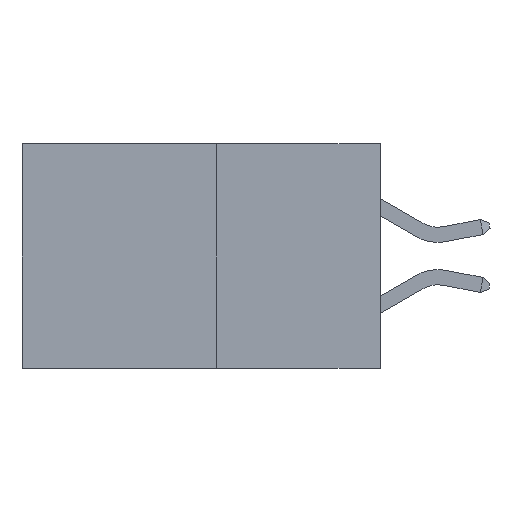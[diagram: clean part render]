
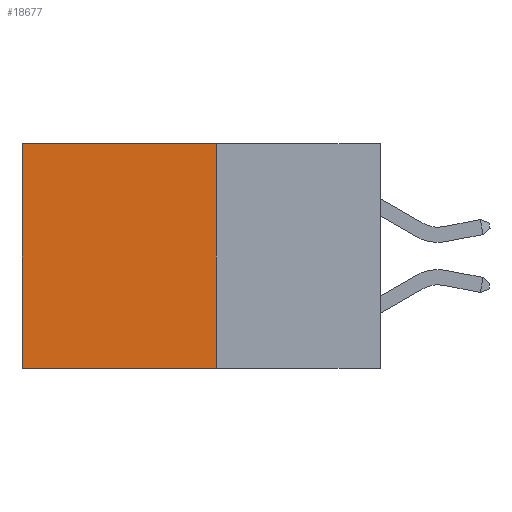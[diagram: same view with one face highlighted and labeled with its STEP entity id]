
A CAD part, left-side view. The second image highlights one B-rep face of the part: STEP entity #18677.
In plain terms, the highlighted planar face has unit normal (-1, 0, 0).
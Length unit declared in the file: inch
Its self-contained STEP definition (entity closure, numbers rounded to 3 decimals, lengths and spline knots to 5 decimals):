
#547 = DIRECTION ( 'NONE',  ( 0., 0., -1. ) ) ;
#1519 = EDGE_CURVE ( 'NONE', #11009, #12221, #9132, .T. ) ;
#2739 = ORIENTED_EDGE ( 'NONE', *, *, #11771, .T. ) ;
#2845 = VERTEX_POINT ( 'NONE', #14549 ) ;
#2988 = EDGE_CURVE ( 'NONE', #18688, #11009, #19466, .T. ) ;
#3750 = ORIENTED_EDGE ( 'NONE', *, *, #1519, .F. ) ;
#3765 = VECTOR ( 'NONE', #15501, 39.37008 ) ;
#4001 = AXIS2_PLACEMENT_3D ( 'NONE', #19031, #20812, #10051 ) ;
#4992 = FACE_OUTER_BOUND ( 'NONE', #12676, .T. ) ;
#8182 = VECTOR ( 'NONE', #547, 39.37008 ) ;
#9132 = LINE ( 'NONE', #15919, #3765 ) ;
#9325 = LINE ( 'NONE', #14855, #8182 ) ;
#9678 = CARTESIAN_POINT ( 'NONE',  ( 0.277, 0.27, -0.37 ) ) ;
#9979 = DIRECTION ( 'NONE',  ( 0., 0., -1. ) ) ;
#10051 = DIRECTION ( 'NONE',  ( 0., 0., -1. ) ) ;
#11009 = VERTEX_POINT ( 'NONE', #20145 ) ;
#11771 = EDGE_CURVE ( 'NONE', #2845, #12221, #9325, .T. ) ;
#11930 = CARTESIAN_POINT ( 'NONE',  ( 0.277, 0.27, 0. ) ) ;
#12221 = VERTEX_POINT ( 'NONE', #12390 ) ;
#12390 = CARTESIAN_POINT ( 'NONE',  ( 0.277, 0.59, -0.37 ) ) ;
#12676 = EDGE_LOOP ( 'NONE', ( #2739, #3750, #13959, #19183 ) ) ;
#13768 = DIRECTION ( 'NONE',  ( 0., 1., 0. ) ) ;
#13932 = VECTOR ( 'NONE', #13768, 39.37008 ) ;
#13959 = ORIENTED_EDGE ( 'NONE', *, *, #2988, .F. ) ;
#14549 = CARTESIAN_POINT ( 'NONE',  ( 0.277, 0.59, 0. ) ) ;
#14715 = EDGE_CURVE ( 'NONE', #18688, #2845, #22304, .T. ) ;
#14855 = CARTESIAN_POINT ( 'NONE',  ( 0.277, 0.59, -0.37 ) ) ;
#15493 = CARTESIAN_POINT ( 'NONE',  ( 0.277, 0.27, 0. ) ) ;
#15501 = DIRECTION ( 'NONE',  ( 0., 1., 0. ) ) ;
#15919 = CARTESIAN_POINT ( 'NONE',  ( 0.277, 0.27, -0.37 ) ) ;
#17213 = PLANE ( 'NONE',  #4001 ) ;
#18677 = ADVANCED_FACE ( 'NONE', ( #4992 ), #17213, .F. ) ;
#18688 = VERTEX_POINT ( 'NONE', #15493 ) ;
#19031 = CARTESIAN_POINT ( 'NONE',  ( 0.277, 0.27, -0.37 ) ) ;
#19183 = ORIENTED_EDGE ( 'NONE', *, *, #14715, .T. ) ;
#19466 = LINE ( 'NONE', #9678, #20046 ) ;
#20046 = VECTOR ( 'NONE', #9979, 39.37008 ) ;
#20145 = CARTESIAN_POINT ( 'NONE',  ( 0.277, 0.27, -0.37 ) ) ;
#20812 = DIRECTION ( 'NONE',  ( 1., 0., 0. ) ) ;
#22304 = LINE ( 'NONE', #11930, #13932 ) ;
